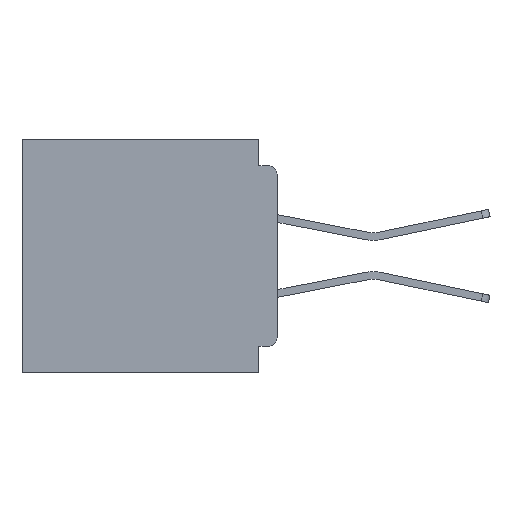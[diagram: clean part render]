
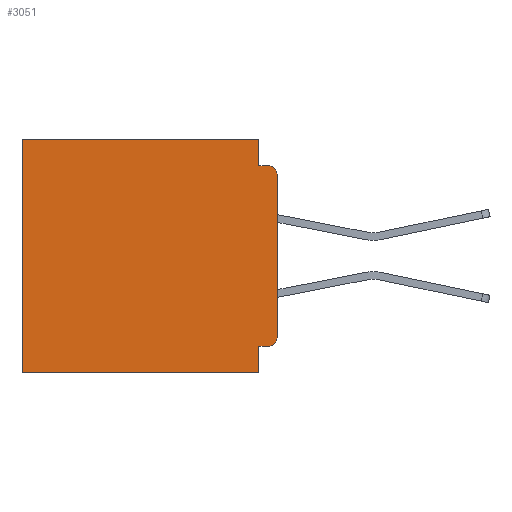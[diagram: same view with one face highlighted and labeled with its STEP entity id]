
A CAD part, left-side view. The second image highlights one B-rep face of the part: STEP entity #3051.
In plain terms, the highlighted planar face has unit normal (-1, 0, 0).
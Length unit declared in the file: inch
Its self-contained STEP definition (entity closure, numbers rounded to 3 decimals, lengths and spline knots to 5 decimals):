
#239 = VECTOR ( 'NONE', #29329, 39.37008 ) ;
#610 = EDGE_CURVE ( 'NONE', #17331, #33946, #21466, .T. ) ;
#1652 = EDGE_CURVE ( 'NONE', #24461, #29613, #32309, .T. ) ;
#2805 = LINE ( 'NONE', #30902, #35473 ) ;
#3051 = ADVANCED_FACE ( 'NONE', ( #9749 ), #7191, .F. ) ;
#3160 = CARTESIAN_POINT ( 'NONE',  ( 0.3, 0., 0. ) ) ;
#4044 = EDGE_CURVE ( 'NONE', #20146, #12366, #6666, .T. ) ;
#4345 = DIRECTION ( 'NONE',  ( 0., 1., 0. ) ) ;
#6270 = CARTESIAN_POINT ( 'NONE',  ( 0.3, 0., -0.4 ) ) ;
#6379 = ORIENTED_EDGE ( 'NONE', *, *, #1652, .F. ) ;
#6666 = LINE ( 'NONE', #29497, #22443 ) ;
#6734 = CARTESIAN_POINT ( 'NONE',  ( 0.3, 0.031, -0.355 ) ) ;
#7191 = PLANE ( 'NONE',  #39469 ) ;
#7840 = VECTOR ( 'NONE', #9809, 39.37008 ) ;
#7883 = EDGE_CURVE ( 'NONE', #12366, #25602, #16250, .T. ) ;
#8798 = DIRECTION ( 'NONE',  ( 0., 0., -1. ) ) ;
#8873 = CARTESIAN_POINT ( 'NONE',  ( 0.3, 0.015, -0.34 ) ) ;
#8918 = DIRECTION ( 'NONE',  ( 0., 0., -1. ) ) ;
#8960 = EDGE_CURVE ( 'NONE', #37777, #29613, #40495, .T. ) ;
#9749 = FACE_OUTER_BOUND ( 'NONE', #12142, .T. ) ;
#9809 = DIRECTION ( 'NONE',  ( 0., 1., 0. ) ) ;
#9953 = EDGE_CURVE ( 'NONE', #17331, #20486, #2805, .T. ) ;
#10202 = DIRECTION ( 'NONE',  ( -1., 0., 0. ) ) ;
#10602 = ORIENTED_EDGE ( 'NONE', *, *, #9953, .F. ) ;
#11031 = AXIS2_PLACEMENT_3D ( 'NONE', #29095, #10202, #32296 ) ;
#12106 = DIRECTION ( 'NONE',  ( 0., 0., -1. ) ) ;
#12142 = EDGE_LOOP ( 'NONE', ( #6379, #12836, #20881, #10602, #24410, #17758, #19810, #18372, #39307, #15855 ) ) ;
#12366 = VERTEX_POINT ( 'NONE', #17448 ) ;
#12381 = CARTESIAN_POINT ( 'NONE',  ( 0.3, 0.015, -0.355 ) ) ;
#12836 = ORIENTED_EDGE ( 'NONE', *, *, #13590, .T. ) ;
#13283 = CARTESIAN_POINT ( 'NONE',  ( 0.3, 0.437, 0. ) ) ;
#13590 = EDGE_CURVE ( 'NONE', #24461, #14815, #35160, .T. ) ;
#14815 = VERTEX_POINT ( 'NONE', #15778 ) ;
#15747 = DIRECTION ( 'NONE',  ( 1., 0., 0. ) ) ;
#15778 = CARTESIAN_POINT ( 'NONE',  ( 0.3, 0.015, -0.045 ) ) ;
#15855 = ORIENTED_EDGE ( 'NONE', *, *, #8960, .T. ) ;
#16250 = LINE ( 'NONE', #22313, #7840 ) ;
#17187 = LINE ( 'NONE', #35625, #239 ) ;
#17331 = VERTEX_POINT ( 'NONE', #22495 ) ;
#17448 = CARTESIAN_POINT ( 'NONE',  ( 0.3, 0.031, -0.4 ) ) ;
#17758 = ORIENTED_EDGE ( 'NONE', *, *, #24057, .T. ) ;
#18372 = ORIENTED_EDGE ( 'NONE', *, *, #4044, .F. ) ;
#19810 = ORIENTED_EDGE ( 'NONE', *, *, #7883, .F. ) ;
#20141 = LINE ( 'NONE', #34050, #36405 ) ;
#20146 = VERTEX_POINT ( 'NONE', #6734 ) ;
#20456 = VECTOR ( 'NONE', #4345, 39.37008 ) ;
#20486 = VERTEX_POINT ( 'NONE', #39936 ) ;
#20881 = ORIENTED_EDGE ( 'NONE', *, *, #24521, .F. ) ;
#21466 = LINE ( 'NONE', #3160, #20456 ) ;
#22313 = CARTESIAN_POINT ( 'NONE',  ( 0.3, 0., -0.4 ) ) ;
#22443 = VECTOR ( 'NONE', #29391, 39.37008 ) ;
#22495 = CARTESIAN_POINT ( 'NONE',  ( 0.3, 0.031, 0. ) ) ;
#22633 = DIRECTION ( 'NONE',  ( 0., 0., -1. ) ) ;
#23653 = CARTESIAN_POINT ( 'NONE',  ( 0.3, 0., -0.355 ) ) ;
#24057 = EDGE_CURVE ( 'NONE', #33946, #25602, #20141, .T. ) ;
#24410 = ORIENTED_EDGE ( 'NONE', *, *, #610, .T. ) ;
#24461 = VERTEX_POINT ( 'NONE', #38255 ) ;
#24521 = EDGE_CURVE ( 'NONE', #20486, #14815, #17187, .T. ) ;
#25602 = VERTEX_POINT ( 'NONE', #32307 ) ;
#29095 = CARTESIAN_POINT ( 'NONE',  ( 0.3, 0.015, -0.06 ) ) ;
#29329 = DIRECTION ( 'NONE',  ( 0., -1., 0. ) ) ;
#29391 = DIRECTION ( 'NONE',  ( 0., 0., -1. ) ) ;
#29497 = CARTESIAN_POINT ( 'NONE',  ( 0.3, 0.031, -0.4 ) ) ;
#29613 = VERTEX_POINT ( 'NONE', #31102 ) ;
#30202 = DIRECTION ( 'NONE',  ( 0., 1., 0. ) ) ;
#30902 = CARTESIAN_POINT ( 'NONE',  ( 0.3, 0.031, 0. ) ) ;
#30994 = DIRECTION ( 'NONE',  ( -1., 0., 0. ) ) ;
#31102 = CARTESIAN_POINT ( 'NONE',  ( 0.3, 0., -0.34 ) ) ;
#31790 = EDGE_CURVE ( 'NONE', #37777, #20146, #34066, .T. ) ;
#32296 = DIRECTION ( 'NONE',  ( 0., 0., -1. ) ) ;
#32307 = CARTESIAN_POINT ( 'NONE',  ( 0.3, 0.437, -0.4 ) ) ;
#32309 = LINE ( 'NONE', #32535, #40615 ) ;
#32535 = CARTESIAN_POINT ( 'NONE',  ( 0.3, 0., -0.4 ) ) ;
#32816 = AXIS2_PLACEMENT_3D ( 'NONE', #8873, #30994, #12106 ) ;
#33099 = VECTOR ( 'NONE', #30202, 39.37008 ) ;
#33946 = VERTEX_POINT ( 'NONE', #13283 ) ;
#34050 = CARTESIAN_POINT ( 'NONE',  ( 0.3, 0.437, -0.4 ) ) ;
#34066 = LINE ( 'NONE', #23653, #33099 ) ;
#35160 = CIRCLE ( 'NONE', #11031, 0.015 ) ;
#35473 = VECTOR ( 'NONE', #8918, 39.37008 ) ;
#35625 = CARTESIAN_POINT ( 'NONE',  ( 0.3, 0., -0.045 ) ) ;
#36405 = VECTOR ( 'NONE', #8798, 39.37008 ) ;
#37661 = DIRECTION ( 'NONE',  ( 0., 0., -1. ) ) ;
#37777 = VERTEX_POINT ( 'NONE', #12381 ) ;
#38255 = CARTESIAN_POINT ( 'NONE',  ( 0.3, 0., -0.06 ) ) ;
#39307 = ORIENTED_EDGE ( 'NONE', *, *, #31790, .F. ) ;
#39469 = AXIS2_PLACEMENT_3D ( 'NONE', #6270, #15747, #22633 ) ;
#39936 = CARTESIAN_POINT ( 'NONE',  ( 0.3, 0.031, -0.045 ) ) ;
#40495 = CIRCLE ( 'NONE', #32816, 0.015 ) ;
#40615 = VECTOR ( 'NONE', #37661, 39.37008 ) ;
